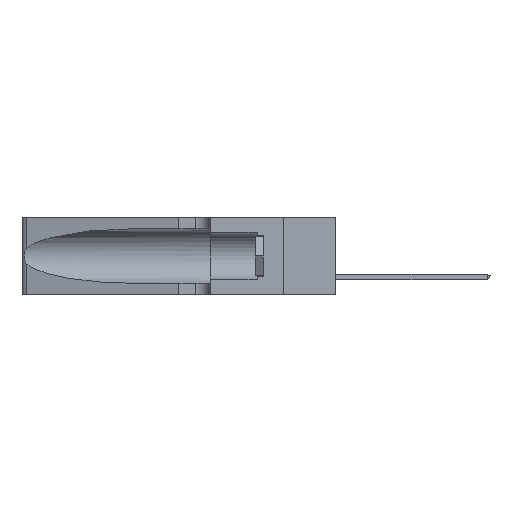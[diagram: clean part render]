
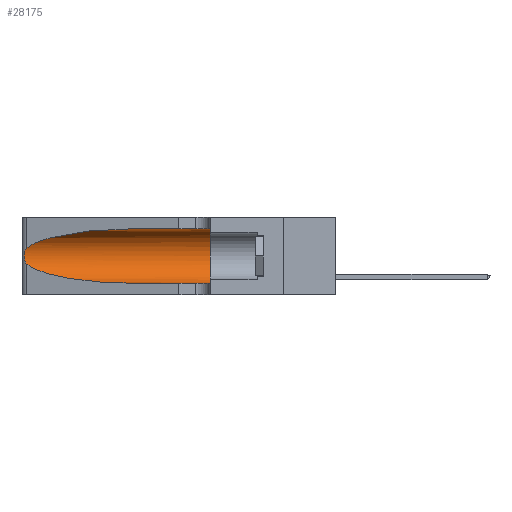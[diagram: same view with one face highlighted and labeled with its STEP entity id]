
A CAD part, left-side view. The second image highlights one B-rep face of the part: STEP entity #28175.
In plain terms, the highlighted cylindrical face has radius 3.308 mm (diameter 6.617 mm), a partial arc.
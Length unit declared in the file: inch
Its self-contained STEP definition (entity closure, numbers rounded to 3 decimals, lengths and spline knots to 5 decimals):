
#898 = ORIENTED_EDGE ( 'NONE', *, *, #27907, .T. ) ;
#1093 = EDGE_CURVE ( 'NONE', #40997, #36568, #36937, .T. ) ;
#2121 = CARTESIAN_POINT ( 'NONE',  ( 0.2373, 1.15595, 0.28018 ) ) ;
#2483 = CARTESIAN_POINT ( 'NONE',  ( 0.26075, 1.23896, 0.19203 ) ) ;
#2828 = CARTESIAN_POINT ( 'NONE',  ( 0.25854, 1.2359, 0.20912 ) ) ;
#4919 = CARTESIAN_POINT ( 'NONE',  ( 0.25487, 1.22718, 0.14631 ) ) ;
#5230 = CARTESIAN_POINT ( 'NONE',  ( 0.1305, 1.61858, 0.31525 ) ) ;
#5979 = VECTOR ( 'NONE', #31769, 39.37008 ) ;
#6907 = CARTESIAN_POINT ( 'NONE',  ( 0.26075, 1.23896, 0.178 ) ) ;
#8211 = CARTESIAN_POINT ( 'NONE',  ( 0.2373, 1.15595, 0.08982 ) ) ;
#9165 = CARTESIAN_POINT ( 'NONE',  ( 0.1305, 0.72297, 0.05475 ) ) ;
#10475 = CARTESIAN_POINT ( 'NONE',  ( 0.25555, 1.22994, 0.2215 ) ) ;
#11124 = ORIENTED_EDGE ( 'NONE', *, *, #1093, .F. ) ;
#13885 = CARTESIAN_POINT ( 'NONE',  ( 0.25487, 1.22718, 0.22369 ) ) ;
#14962 = B_SPLINE_CURVE_WITH_KNOTS ( 'NONE', 3,
 ( #21684, #10475, #37755, #29738, #2828, #49328, #2483, #6907, #29544, #37930, #37574, #45400, #49498, #30089 ),
 .UNSPECIFIED., .F., .F.,
 ( 4, 2, 2, 2, 2, 2, 4 ),
 ( 0., 0.00027, 0.00053, 0.00107, 0.0016, 0.00187, 0.00214 ),
 .UNSPECIFIED. ) ;
#14977 = EDGE_CURVE ( 'NONE', #40216, #23619, #34706, .T. ) ;
#16284 = CARTESIAN_POINT ( 'NONE',  ( 0.1305, 0.72297, 0.05475 ) ) ;
#19154 = CARTESIAN_POINT ( 'NONE',  ( 0.25487, 1.22718, 0.14631 ) ) ;
#19457 = DIRECTION ( 'NONE',  ( 0., 1., 0. ) ) ;
#20416 = CYLINDRICAL_SURFACE ( 'NONE', #30438, 0.13025 ) ;
#20662 = CARTESIAN_POINT ( 'NONE',  ( 0.1305, 0.72297, 0.31525 ) ) ;
#20820 = VERTEX_POINT ( 'NONE', #27198 ) ;
#21040 = CIRCLE ( 'NONE', #21272, 0.13025 ) ;
#21272 = AXIS2_PLACEMENT_3D ( 'NONE', #50368, #19457, #27796 ) ;
#21684 = CARTESIAN_POINT ( 'NONE',  ( 0.25487, 1.22718, 0.22369 ) ) ;
#22403 = FACE_OUTER_BOUND ( 'NONE', #44490, .T. ) ;
#22758 = ORIENTED_EDGE ( 'NONE', *, *, #14977, .T. ) ;
#23619 = VERTEX_POINT ( 'NONE', #32770 ) ;
#25463 = CARTESIAN_POINT ( 'NONE',  ( 0.1305, 0.72297, 0.31525 ) ) ;
#27198 = CARTESIAN_POINT ( 'NONE',  ( 0.25487, 1.22718, 0.22369 ) ) ;
#27796 = DIRECTION ( 'NONE',  ( 0., 0., 1. ) ) ;
#27907 = EDGE_CURVE ( 'NONE', #28176, #40216, #36108, .T. ) ;
#28175 = ADVANCED_FACE ( 'NONE', ( #22403 ), #20416, .F. ) ;
#28176 = VERTEX_POINT ( 'NONE', #19154 ) ;
#29544 = CARTESIAN_POINT ( 'NONE',  ( 0.26017, 1.23833, 0.17102 ) ) ;
#29738 = CARTESIAN_POINT ( 'NONE',  ( 0.25787, 1.23484, 0.2124 ) ) ;
#29777 = DIRECTION ( 'NONE',  ( 0., -1., 0. ) ) ;
#30089 = CARTESIAN_POINT ( 'NONE',  ( 0.25487, 1.22718, 0.14631 ) ) ;
#30438 = AXIS2_PLACEMENT_3D ( 'NONE', #40939, #29777, #38441 ) ;
#31472 =( BOUNDED_CURVE ( )  B_SPLINE_CURVE ( 3, ( #25463, #37053, #2121, #13885 ),
 .UNSPECIFIED., .F., .T. ) 
 B_SPLINE_CURVE_WITH_KNOTS ( ( 4, 4 ),
 ( 1.5708, 2.84003 ),
 .UNSPECIFIED. ) 
 CURVE ( )  GEOMETRIC_REPRESENTATION_ITEM ( )  RATIONAL_B_SPLINE_CURVE ( ( 1., 0.87, 0.87, 1. ) ) 
 REPRESENTATION_ITEM ( '' )  );
#31769 = DIRECTION ( 'NONE',  ( 0., -1., 0. ) ) ;
#32770 = CARTESIAN_POINT ( 'NONE',  ( 0.1305, 0.35, 0.05475 ) ) ;
#34706 = LINE ( 'NONE', #38952, #5979 ) ;
#36108 =( BOUNDED_CURVE ( )  B_SPLINE_CURVE ( 3, ( #4919, #8211, #39382, #9165 ),
 .UNSPECIFIED., .F., .T. ) 
 B_SPLINE_CURVE_WITH_KNOTS ( ( 4, 4 ),
 ( 3.44316, 4.71239 ),
 .UNSPECIFIED. ) 
 CURVE ( )  GEOMETRIC_REPRESENTATION_ITEM ( )  RATIONAL_B_SPLINE_CURVE ( ( 1., 0.87, 0.87, 1. ) ) 
 REPRESENTATION_ITEM ( '' )  );
#36340 = VECTOR ( 'NONE', #36453, 39.37008 ) ;
#36453 = DIRECTION ( 'NONE',  ( 0., -1., 0. ) ) ;
#36568 = VERTEX_POINT ( 'NONE', #37232 ) ;
#36937 = LINE ( 'NONE', #5230, #36340 ) ;
#37053 = CARTESIAN_POINT ( 'NONE',  ( 0.18966, 0.96281, 0.31525 ) ) ;
#37232 = CARTESIAN_POINT ( 'NONE',  ( 0.1305, 0.35, 0.31525 ) ) ;
#37355 = EDGE_CURVE ( 'NONE', #20820, #28176, #14962, .T. ) ;
#37574 = CARTESIAN_POINT ( 'NONE',  ( 0.25789, 1.23486, 0.15765 ) ) ;
#37755 = CARTESIAN_POINT ( 'NONE',  ( 0.25639, 1.23184, 0.21858 ) ) ;
#37930 = CARTESIAN_POINT ( 'NONE',  ( 0.25856, 1.23593, 0.16098 ) ) ;
#38052 = ORIENTED_EDGE ( 'NONE', *, *, #45565, .T. ) ;
#38441 = DIRECTION ( 'NONE',  ( 0., 0., -1. ) ) ;
#38952 = CARTESIAN_POINT ( 'NONE',  ( 0.1305, 1.61858, 0.05475 ) ) ;
#39382 = CARTESIAN_POINT ( 'NONE',  ( 0.18966, 0.96281, 0.05475 ) ) ;
#40216 = VERTEX_POINT ( 'NONE', #16284 ) ;
#40939 = CARTESIAN_POINT ( 'NONE',  ( 0.1305, 1.61858, 0.185 ) ) ;
#40997 = VERTEX_POINT ( 'NONE', #20662 ) ;
#42924 = EDGE_CURVE ( 'NONE', #36568, #23619, #21040, .T. ) ;
#43909 = ORIENTED_EDGE ( 'NONE', *, *, #37355, .T. ) ;
#44490 = EDGE_LOOP ( 'NONE', ( #38052, #43909, #898, #22758, #46575, #11124 ) ) ;
#45400 = CARTESIAN_POINT ( 'NONE',  ( 0.25639, 1.23186, 0.15144 ) ) ;
#45565 = EDGE_CURVE ( 'NONE', #40997, #20820, #31472, .T. ) ;
#46575 = ORIENTED_EDGE ( 'NONE', *, *, #42924, .F. ) ;
#49328 = CARTESIAN_POINT ( 'NONE',  ( 0.26018, 1.23835, 0.19895 ) ) ;
#49498 = CARTESIAN_POINT ( 'NONE',  ( 0.25555, 1.22993, 0.14849 ) ) ;
#50368 = CARTESIAN_POINT ( 'NONE',  ( 0.1305, 0.35, 0.185 ) ) ;
